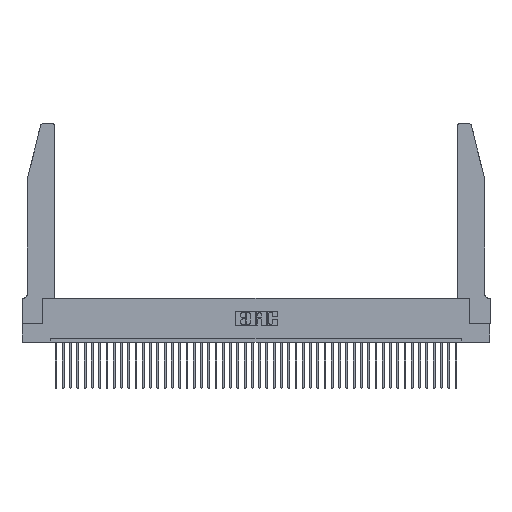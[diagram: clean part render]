
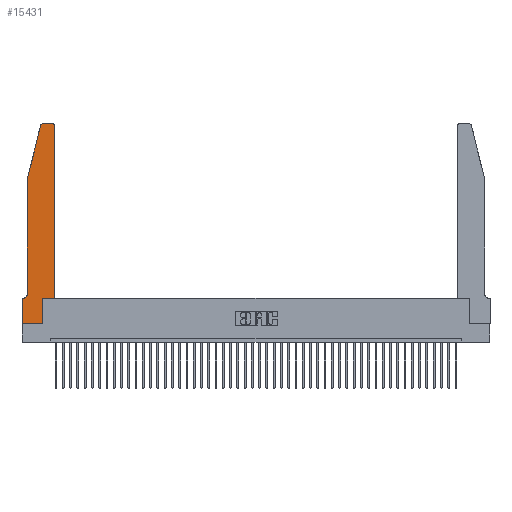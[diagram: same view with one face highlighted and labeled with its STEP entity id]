
A CAD part, top view. The second image highlights one B-rep face of the part: STEP entity #15431.
In plain terms, the highlighted planar face has unit normal (0, 0, 1).
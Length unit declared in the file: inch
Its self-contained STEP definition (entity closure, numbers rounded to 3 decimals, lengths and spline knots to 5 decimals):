
#127 = CARTESIAN_POINT ( 'NONE',  ( 0.4505, 0.35, 0.37 ) ) ;
#1083 = VERTEX_POINT ( 'NONE', #24382 ) ;
#1647 = ORIENTED_EDGE ( 'NONE', *, *, #31140, .T. ) ;
#2583 = DIRECTION ( 'NONE',  ( 0., 0., -1. ) ) ;
#2729 = DIRECTION ( 'NONE',  ( -1., 0., 0. ) ) ;
#2959 = EDGE_CURVE ( 'NONE', #5157, #1083, #29415, .T. ) ;
#3012 = CARTESIAN_POINT ( 'NONE',  ( 0., 0.35, 0.37 ) ) ;
#3644 = EDGE_CURVE ( 'NONE', #11158, #16048, #27728, .T. ) ;
#3938 = VECTOR ( 'NONE', #27905, 39.37008 ) ;
#4036 = CARTESIAN_POINT ( 'NONE',  ( 0.4505, 0.35, 0.37 ) ) ;
#4489 = VECTOR ( 'NONE', #10517, 39.37008 ) ;
#5157 = VERTEX_POINT ( 'NONE', #9387 ) ;
#5478 = EDGE_CURVE ( 'NONE', #35046, #43623, #38297, .T. ) ;
#5583 = LINE ( 'NONE', #34467, #3938 ) ;
#5700 = PLANE ( 'NONE',  #29428 ) ;
#5857 = VECTOR ( 'NONE', #31753, 39.37008 ) ;
#6724 = LINE ( 'NONE', #41389, #4489 ) ;
#7036 = DIRECTION ( 'NONE',  ( 1., 0., 0. ) ) ;
#7152 = AXIS2_PLACEMENT_3D ( 'NONE', #21628, #7673, #7530 ) ;
#7530 = DIRECTION ( 'NONE',  ( 1., 0., 0. ) ) ;
#7673 = DIRECTION ( 'NONE',  ( 0., 0., 1. ) ) ;
#7834 = VERTEX_POINT ( 'NONE', #25778 ) ;
#8724 = EDGE_CURVE ( 'NONE', #15935, #7834, #39557, .T. ) ;
#9387 = CARTESIAN_POINT ( 'NONE',  ( 0.4505, 2.72, 0.37 ) ) ;
#9532 = CARTESIAN_POINT ( 'NONE',  ( 0.2865, 0.35, 0.37 ) ) ;
#10517 = DIRECTION ( 'NONE',  ( -1., 0., 0. ) ) ;
#11158 = VERTEX_POINT ( 'NONE', #28726 ) ;
#11968 = DIRECTION ( 'NONE',  ( 0., -1., 0. ) ) ;
#13220 = CARTESIAN_POINT ( 'NONE',  ( 0.4505, 0.35, 0.37 ) ) ;
#14066 = AXIS2_PLACEMENT_3D ( 'NONE', #30439, #2583, #2729 ) ;
#14454 = LINE ( 'NONE', #13220, #21997 ) ;
#14911 = ORIENTED_EDGE ( 'NONE', *, *, #38003, .T. ) ;
#15431 = ADVANCED_FACE ( 'NONE', ( #25123 ), #5700, .T. ) ;
#15925 = DIRECTION ( 'NONE',  ( 0., 0., 1. ) ) ;
#15935 = VERTEX_POINT ( 'NONE', #36194 ) ;
#16034 = LINE ( 'NONE', #20972, #35040 ) ;
#16048 = VERTEX_POINT ( 'NONE', #43155 ) ;
#16059 = ORIENTED_EDGE ( 'NONE', *, *, #21505, .T. ) ;
#16545 = CARTESIAN_POINT ( 'NONE',  ( 0.0755, 0.42, 0.37 ) ) ;
#16977 = CARTESIAN_POINT ( 'NONE',  ( 0., 0., 0.37 ) ) ;
#18282 = ORIENTED_EDGE ( 'NONE', *, *, #35797, .T. ) ;
#18331 = DIRECTION ( 'NONE',  ( 0., 1., 0. ) ) ;
#18910 = CARTESIAN_POINT ( 'NONE',  ( 0.0755, 2., 0.37 ) ) ;
#19575 = DIRECTION ( 'NONE',  ( 1., 0., 0. ) ) ;
#20972 = CARTESIAN_POINT ( 'NONE',  ( 0.2605, 2.75, 0.37 ) ) ;
#21505 = EDGE_CURVE ( 'NONE', #30063, #35046, #6724, .T. ) ;
#21628 = CARTESIAN_POINT ( 'NONE',  ( 0.284, 2.72, 0.37 ) ) ;
#21684 = VECTOR ( 'NONE', #18331, 39.37008 ) ;
#21997 = VECTOR ( 'NONE', #30734, 39.37008 ) ;
#22163 = ORIENTED_EDGE ( 'NONE', *, *, #26215, .T. ) ;
#22188 = AXIS2_PLACEMENT_3D ( 'NONE', #33612, #15925, #19575 ) ;
#23590 = CARTESIAN_POINT ( 'NONE',  ( 0., 0., 0.37 ) ) ;
#23698 = EDGE_CURVE ( 'NONE', #28947, #15935, #28690, .T. ) ;
#24382 = CARTESIAN_POINT ( 'NONE',  ( 0.4205, 2.75, 0.37 ) ) ;
#24488 = EDGE_LOOP ( 'NONE', ( #1647, #27635, #31645, #33970, #34539, #16059, #28935, #22163, #29908, #14911, #18282, #39381 ) ) ;
#25045 = EDGE_CURVE ( 'NONE', #7834, #39562, #35102, .T. ) ;
#25123 = FACE_OUTER_BOUND ( 'NONE', #24488, .T. ) ;
#25778 = CARTESIAN_POINT ( 'NONE',  ( 0.0755, 2., 0.37 ) ) ;
#26215 = EDGE_CURVE ( 'NONE', #43623, #11158, #5583, .T. ) ;
#27635 = ORIENTED_EDGE ( 'NONE', *, *, #23698, .T. ) ;
#27728 = LINE ( 'NONE', #9532, #31021 ) ;
#27809 = CIRCLE ( 'NONE', #14066, 0.07 ) ;
#27905 = DIRECTION ( 'NONE',  ( 1., 0., 0. ) ) ;
#28112 = VERTEX_POINT ( 'NONE', #4036 ) ;
#28690 = CIRCLE ( 'NONE', #7152, 0.03 ) ;
#28726 = CARTESIAN_POINT ( 'NONE',  ( 0.2865, 0., 0.37 ) ) ;
#28935 = ORIENTED_EDGE ( 'NONE', *, *, #5478, .T. ) ;
#28947 = VERTEX_POINT ( 'NONE', #32684 ) ;
#29042 = VECTOR ( 'NONE', #37388, 39.37008 ) ;
#29415 = CIRCLE ( 'NONE', #22188, 0.03 ) ;
#29428 = AXIS2_PLACEMENT_3D ( 'NONE', #40988, #33720, #7036 ) ;
#29660 = VECTOR ( 'NONE', #11968, 39.37008 ) ;
#29908 = ORIENTED_EDGE ( 'NONE', *, *, #3644, .T. ) ;
#30063 = VERTEX_POINT ( 'NONE', #40543 ) ;
#30439 = CARTESIAN_POINT ( 'NONE',  ( 0.0055, 0.42, 0.37 ) ) ;
#30527 = LINE ( 'NONE', #127, #21684 ) ;
#30734 = DIRECTION ( 'NONE',  ( 1., 0., 0. ) ) ;
#31021 = VECTOR ( 'NONE', #33866, 39.37008 ) ;
#31140 = EDGE_CURVE ( 'NONE', #1083, #28947, #16034, .T. ) ;
#31645 = ORIENTED_EDGE ( 'NONE', *, *, #8724, .T. ) ;
#31753 = DIRECTION ( 'NONE',  ( -0.239, -0.971, 0. ) ) ;
#32684 = CARTESIAN_POINT ( 'NONE',  ( 0.284, 2.75, 0.37 ) ) ;
#33612 = CARTESIAN_POINT ( 'NONE',  ( 0.4205, 2.72, 0.37 ) ) ;
#33720 = DIRECTION ( 'NONE',  ( 0., 0., 1. ) ) ;
#33866 = DIRECTION ( 'NONE',  ( 0., 1., 0. ) ) ;
#33970 = ORIENTED_EDGE ( 'NONE', *, *, #25045, .T. ) ;
#34467 = CARTESIAN_POINT ( 'NONE',  ( 0., 0., 0.37 ) ) ;
#34539 = ORIENTED_EDGE ( 'NONE', *, *, #44072, .T. ) ;
#35040 = VECTOR ( 'NONE', #35141, 39.37008 ) ;
#35046 = VERTEX_POINT ( 'NONE', #3012 ) ;
#35102 = LINE ( 'NONE', #18910, #29660 ) ;
#35141 = DIRECTION ( 'NONE',  ( -1., 0., 0. ) ) ;
#35342 = CARTESIAN_POINT ( 'NONE',  ( 0.0755, 2., 0.37 ) ) ;
#35797 = EDGE_CURVE ( 'NONE', #28112, #5157, #30527, .T. ) ;
#36194 = CARTESIAN_POINT ( 'NONE',  ( 0.25487, 2.72718, 0.37 ) ) ;
#37388 = DIRECTION ( 'NONE',  ( 0., -1., 0. ) ) ;
#38003 = EDGE_CURVE ( 'NONE', #16048, #28112, #14454, .T. ) ;
#38297 = LINE ( 'NONE', #16977, #29042 ) ;
#39381 = ORIENTED_EDGE ( 'NONE', *, *, #2959, .T. ) ;
#39557 = LINE ( 'NONE', #35342, #5857 ) ;
#39562 = VERTEX_POINT ( 'NONE', #16545 ) ;
#40543 = CARTESIAN_POINT ( 'NONE',  ( 0.0055, 0.35, 0.37 ) ) ;
#40988 = CARTESIAN_POINT ( 'NONE',  ( 0., 0.35, 0.37 ) ) ;
#41389 = CARTESIAN_POINT ( 'NONE',  ( 0.0755, 0.35, 0.37 ) ) ;
#43155 = CARTESIAN_POINT ( 'NONE',  ( 0.2865, 0.35, 0.37 ) ) ;
#43623 = VERTEX_POINT ( 'NONE', #23590 ) ;
#44072 = EDGE_CURVE ( 'NONE', #39562, #30063, #27809, .T. ) ;
